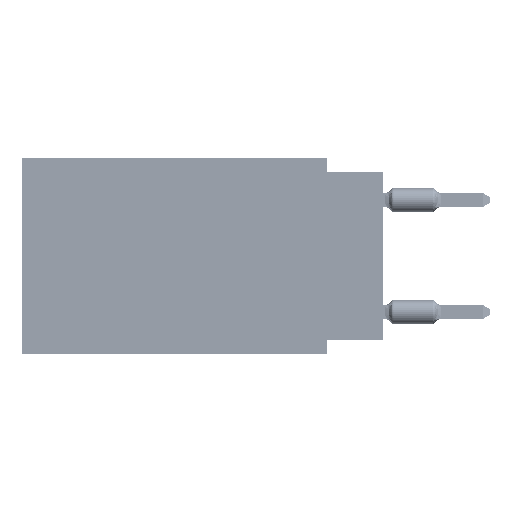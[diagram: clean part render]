
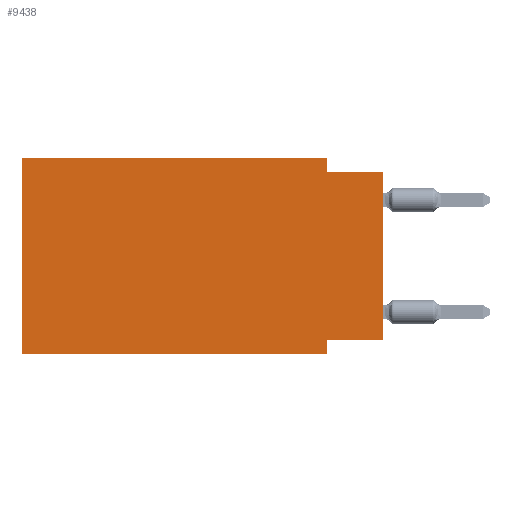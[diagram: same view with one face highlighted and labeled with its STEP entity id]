
A CAD part, left-side view. The second image highlights one B-rep face of the part: STEP entity #9438.
In plain terms, the highlighted planar face has unit normal (-1, 0, 0).
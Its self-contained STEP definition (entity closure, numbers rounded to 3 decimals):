
#1066 = LINE ( 'NONE', #23850, #11364 ) ;
#1885 = EDGE_CURVE ( 'NONE', #67619, #42503, #41859, .T. ) ;
#2665 = VECTOR ( 'NONE', #22386, 1000. ) ;
#2735 = EDGE_CURVE ( 'NONE', #65166, #65083, #46840, .T. ) ;
#3019 = LINE ( 'NONE', #53814, #64542 ) ;
#4017 = CARTESIAN_POINT ( 'NONE',  ( 0., 16.383, -8.89 ) ) ;
#4962 = DIRECTION ( 'NONE',  ( 0., -1., 0. ) ) ;
#4974 = CARTESIAN_POINT ( 'NONE',  ( 0., 2.54, 0. ) ) ;
#5443 = VERTEX_POINT ( 'NONE', #23896 ) ;
#7495 = ORIENTED_EDGE ( 'NONE', *, *, #31217, .F. ) ;
#7980 = DIRECTION ( 'NONE',  ( 0., 0., 1. ) ) ;
#9438 = ADVANCED_FACE ( 'NONE', ( #54796 ), #26056, .F. ) ;
#10566 = CARTESIAN_POINT ( 'NONE',  ( 0., 16.383, -8.89 ) ) ;
#10767 = VERTEX_POINT ( 'NONE', #4017 ) ;
#11083 = VERTEX_POINT ( 'NONE', #21479 ) ;
#11364 = VECTOR ( 'NONE', #14109, 1000. ) ;
#12190 = ORIENTED_EDGE ( 'NONE', *, *, #54056, .F. ) ;
#12884 = DIRECTION ( 'NONE',  ( 0., 0., -1. ) ) ;
#14109 = DIRECTION ( 'NONE',  ( 0., 1., 0. ) ) ;
#15212 = DIRECTION ( 'NONE',  ( 1., 0., 0. ) ) ;
#17598 = CARTESIAN_POINT ( 'NONE',  ( 0., 0., -0.635 ) ) ;
#19804 = CARTESIAN_POINT ( 'NONE',  ( 0., 16.383, 0. ) ) ;
#20362 = CARTESIAN_POINT ( 'NONE',  ( 0., 0., -0.635 ) ) ;
#20506 = EDGE_CURVE ( 'NONE', #10767, #23448, #44908, .T. ) ;
#21180 = CARTESIAN_POINT ( 'NONE',  ( 0., 16.383, 0. ) ) ;
#21479 = CARTESIAN_POINT ( 'NONE',  ( 0., 2.54, -0.635 ) ) ;
#22386 = DIRECTION ( 'NONE',  ( 0., 0., 1. ) ) ;
#23448 = VERTEX_POINT ( 'NONE', #42789 ) ;
#23714 = LINE ( 'NONE', #24450, #48195 ) ;
#23850 = CARTESIAN_POINT ( 'NONE',  ( 0., 0., -8.255 ) ) ;
#23896 = CARTESIAN_POINT ( 'NONE',  ( 0., 2.54, -8.255 ) ) ;
#24195 = ORIENTED_EDGE ( 'NONE', *, *, #57172, .F. ) ;
#24450 = CARTESIAN_POINT ( 'NONE',  ( 0., 2.54, 0. ) ) ;
#26056 = PLANE ( 'NONE',  #46179 ) ;
#26108 = ORIENTED_EDGE ( 'NONE', *, *, #1885, .F. ) ;
#26417 = DIRECTION ( 'NONE',  ( 0., 0., -1. ) ) ;
#28631 = CARTESIAN_POINT ( 'NONE',  ( 0., 0., 0. ) ) ;
#30770 = ORIENTED_EDGE ( 'NONE', *, *, #41075, .F. ) ;
#31217 = EDGE_CURVE ( 'NONE', #65166, #5443, #1066, .T. ) ;
#31409 = DIRECTION ( 'NONE',  ( 0., 0., -1. ) ) ;
#32668 = LINE ( 'NONE', #20362, #69057 ) ;
#33213 = CARTESIAN_POINT ( 'NONE',  ( 0., 16.383, 0. ) ) ;
#36035 = EDGE_CURVE ( 'NONE', #11083, #65083, #32668, .T. ) ;
#40360 = ORIENTED_EDGE ( 'NONE', *, *, #20506, .T. ) ;
#41075 = EDGE_CURVE ( 'NONE', #42503, #11083, #23714, .T. ) ;
#41843 = VECTOR ( 'NONE', #57557, 1000. ) ;
#41859 = LINE ( 'NONE', #45999, #41843 ) ;
#42503 = VERTEX_POINT ( 'NONE', #4974 ) ;
#42789 = CARTESIAN_POINT ( 'NONE',  ( 0., 2.54, -8.89 ) ) ;
#44908 = LINE ( 'NONE', #10566, #52136 ) ;
#45999 = CARTESIAN_POINT ( 'NONE',  ( 0., 16.383, 0. ) ) ;
#46179 = AXIS2_PLACEMENT_3D ( 'NONE', #21180, #15212, #26417 ) ;
#46840 = LINE ( 'NONE', #28631, #51643 ) ;
#48195 = VECTOR ( 'NONE', #12884, 1000. ) ;
#49122 = DIRECTION ( 'NONE',  ( 0., -1., 0. ) ) ;
#50455 = ORIENTED_EDGE ( 'NONE', *, *, #36035, .F. ) ;
#51643 = VECTOR ( 'NONE', #7980, 1000. ) ;
#52136 = VECTOR ( 'NONE', #4962, 1000. ) ;
#53814 = CARTESIAN_POINT ( 'NONE',  ( 0., 2.54, -8.89 ) ) ;
#54056 = EDGE_CURVE ( 'NONE', #5443, #23448, #3019, .T. ) ;
#54796 = FACE_OUTER_BOUND ( 'NONE', #62782, .T. ) ;
#57172 = EDGE_CURVE ( 'NONE', #10767, #67619, #73147, .T. ) ;
#57557 = DIRECTION ( 'NONE',  ( 0., -1., 0. ) ) ;
#57897 = CARTESIAN_POINT ( 'NONE',  ( 0., 0., -8.255 ) ) ;
#62782 = EDGE_LOOP ( 'NONE', ( #68892, #50455, #30770, #26108, #24195, #40360, #12190, #7495 ) ) ;
#64542 = VECTOR ( 'NONE', #31409, 1000. ) ;
#65083 = VERTEX_POINT ( 'NONE', #17598 ) ;
#65166 = VERTEX_POINT ( 'NONE', #57897 ) ;
#67619 = VERTEX_POINT ( 'NONE', #19804 ) ;
#68892 = ORIENTED_EDGE ( 'NONE', *, *, #2735, .T. ) ;
#69057 = VECTOR ( 'NONE', #49122, 1000. ) ;
#73147 = LINE ( 'NONE', #33213, #2665 ) ;
